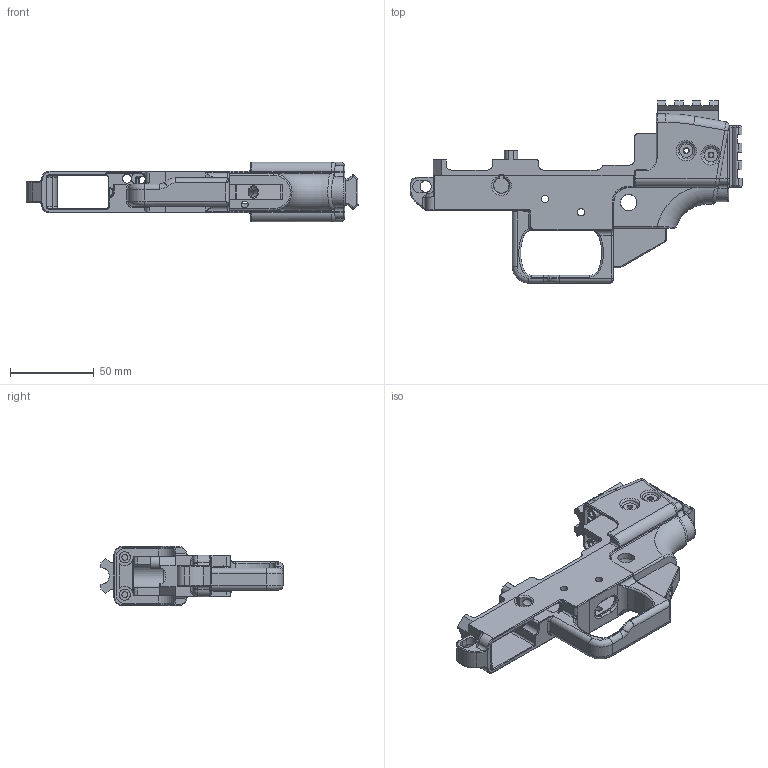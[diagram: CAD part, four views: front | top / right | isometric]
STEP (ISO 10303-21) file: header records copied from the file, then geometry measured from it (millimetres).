
FILE_DESCRIPTION(/* description */ (''),/* implementation_level */ '2;1');
FILE_NAME(/* name */ 'VZ61 Skorpion AR Trigger v15.step',/* time_stamp */ '2020-10-10T01:43:09-04:00',/* author */ (''),/* organization */ (''),/* preprocessor_version */ 'ST-DEVELOPER v18.1',/* originating_system */ 'Autodesk Translation Framework v9.3.0.1241',/* authorisation */ '');
FILE_SCHEMA (('AUTOMOTIVE_DESIGN { 1 0 10303 214 3 1 1 }'));
Length unit declared in the file: millimetre
Products named in the file (5): VZ61 Skorpion AR Trigger; Default; Adapters; Angled Plate; 90 Degree
Assembly tree (4 placements, depth 4):
  VZ61 Skorpion AR Trigger
    Default
    Adapters
      Angled Plate
        90 Degree
Bounding box: 198.2 x 108.81 x 35.48 mm (x, y, z)
Volume: 139871.3 mm3; surface area: 57921.5 mm2
Topology: 4 solids, 4 shells, 707 faces, 1821 edges, 1104 vertices
Faces by surface type: cylinder 265, plane 241, torus 106, bspline 72, sphere 13, cone 10
Full cylindrical faces by diameter (mm): 2.946 x1, 3 x7, 3.5 x1, 3.556 x2, 4 x1, 4.35 x4, 5.461 x1, 5.5 x1, 6.75 x1, 9.85 x2, 27 x1, 27.5 x1
Entity records: 27169 total; most frequent: CARTESIAN_POINT 9853, DIRECTION 3660, ORIENTED_EDGE 3618, EDGE_CURVE 1809, AXIS2_PLACEMENT_3D 1388, VERTEX_POINT 1103, LINE 884, VECTOR 884
